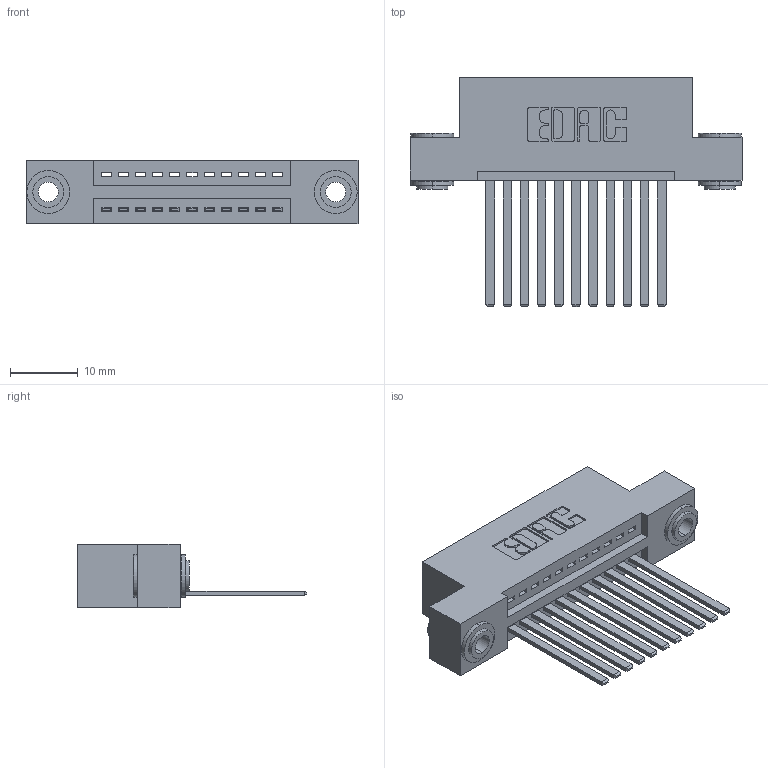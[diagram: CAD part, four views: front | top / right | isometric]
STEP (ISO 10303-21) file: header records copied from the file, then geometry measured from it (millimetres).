
FILE_DESCRIPTION (( 'STEP AP203' ), '1' );
FILE_NAME ('345-011-544-103.STEP', '2019-10-04T00:21:34', ( '' ), ( '' ), 'SwSTEP 2.0', 'SolidWorks 2016', '' );
FILE_SCHEMA (( 'CONFIG_CONTROL_DESIGN' ));
Length unit declared in the file: inch
Products named in the file (4): 345 Part_Flush Mounting Lugs - 0.156 Dia-TH; 345-011-544-103; 345-250-002_345-250-002-102; 345-292-001_345-293-144
Assembly tree (14 placements, depth 2):
  345-011-544-103
    345 Part_Flush Mounting Lugs - 0.156 Dia-TH
    345-292-001_345-293-144  x11
    345-250-002_345-250-002-102  x2
Bounding box: 49.15 x 33.96 x 9.4 mm (x, y, z)
Volume: 4561.1 mm3; surface area: 6236.9 mm2
Topology: 14 solids, 14 shells, 736 faces, 2155 edges, 1418 vertices
Faces by surface type: plane 486, cylinder 242, cone 8
Entity records: 12918 total; most frequent: CARTESIAN_POINT 2216, ORIENTED_EDGE 2154, DIRECTION 2009, EDGE_CURVE 1077, LINE 881, VECTOR 881, VERTEX_POINT 714, AXIS2_PLACEMENT_3D 564
